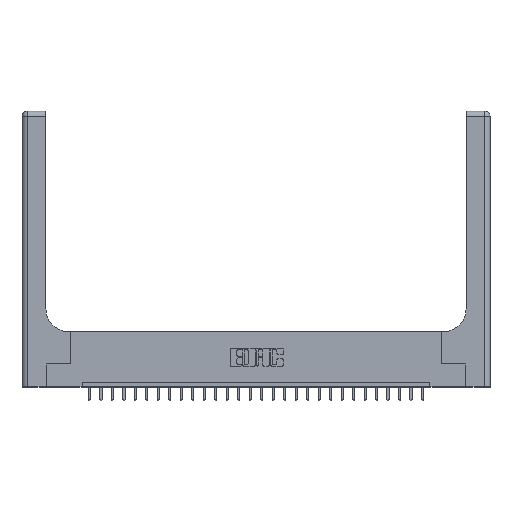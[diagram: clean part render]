
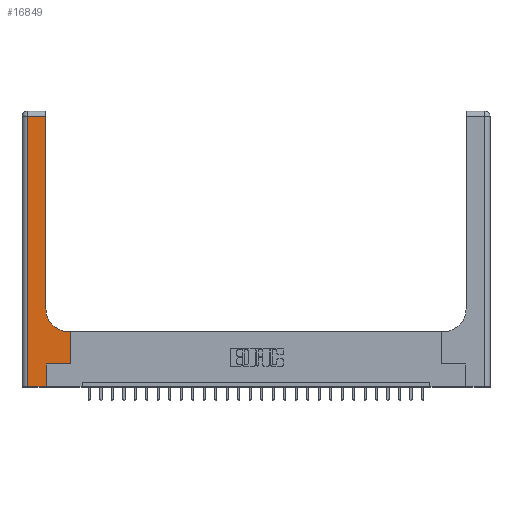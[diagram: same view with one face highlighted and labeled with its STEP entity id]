
A CAD part, top view. The second image highlights one B-rep face of the part: STEP entity #16849.
In plain terms, the highlighted planar face has unit normal (0, 0, 1).
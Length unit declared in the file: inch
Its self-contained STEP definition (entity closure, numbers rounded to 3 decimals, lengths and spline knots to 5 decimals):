
#453 = AXIS2_PLACEMENT_3D ( 'NONE', #2318, #19704, #15861 ) ;
#462 = VECTOR ( 'NONE', #22440, 39.37008 ) ;
#490 = LINE ( 'NONE', #11564, #20848 ) ;
#494 = CARTESIAN_POINT ( 'NONE',  ( 0.528, 0.25, 0.37 ) ) ;
#795 = CARTESIAN_POINT ( 'NONE',  ( 0., 0., 0.37 ) ) ;
#1180 = CARTESIAN_POINT ( 'NONE',  ( 0.265, 0., 0.37 ) ) ;
#1442 = EDGE_CURVE ( 'NONE', #18089, #23932, #17264, .T. ) ;
#1767 = CARTESIAN_POINT ( 'NONE',  ( 0.06, 2.94, 0.37 ) ) ;
#2318 = CARTESIAN_POINT ( 'NONE',  ( 0.51, 0.85, 0.37 ) ) ;
#3366 = EDGE_CURVE ( 'NONE', #8961, #10507, #22909, .T. ) ;
#4182 = ORIENTED_EDGE ( 'NONE', *, *, #21186, .T. ) ;
#6448 = CARTESIAN_POINT ( 'NONE',  ( 0.265, 0.25, 0.37 ) ) ;
#6802 = CARTESIAN_POINT ( 'NONE',  ( 0.51, 0.6, 0.37 ) ) ;
#7119 = VERTEX_POINT ( 'NONE', #1767 ) ;
#7430 = EDGE_CURVE ( 'NONE', #13938, #24035, #20508, .T. ) ;
#8339 = VECTOR ( 'NONE', #15401, 39.37008 ) ;
#8549 = VERTEX_POINT ( 'NONE', #18905 ) ;
#8961 = VERTEX_POINT ( 'NONE', #15860 ) ;
#8978 = CARTESIAN_POINT ( 'NONE',  ( 0.265, 0.25, 0.37 ) ) ;
#8983 = CARTESIAN_POINT ( 'NONE',  ( 0.26, 3., 0.37 ) ) ;
#9111 = ORIENTED_EDGE ( 'NONE', *, *, #1442, .T. ) ;
#9596 = VECTOR ( 'NONE', #21881, 39.37008 ) ;
#9639 = ORIENTED_EDGE ( 'NONE', *, *, #20046, .T. ) ;
#10222 = CARTESIAN_POINT ( 'NONE',  ( 0.528, 0.6, 0.37 ) ) ;
#10507 = VERTEX_POINT ( 'NONE', #8978 ) ;
#11564 = CARTESIAN_POINT ( 'NONE',  ( 0.26, 0.6, 0.37 ) ) ;
#11586 = LINE ( 'NONE', #795, #462 ) ;
#11776 = EDGE_CURVE ( 'NONE', #24035, #18089, #490, .T. ) ;
#12011 = CARTESIAN_POINT ( 'NONE',  ( 0.26, 0.85, 0.37 ) ) ;
#12581 = DIRECTION ( 'NONE',  ( 0., 1., 0. ) ) ;
#12740 = ORIENTED_EDGE ( 'NONE', *, *, #11776, .T. ) ;
#12906 = ORIENTED_EDGE ( 'NONE', *, *, #16806, .T. ) ;
#13363 = EDGE_LOOP ( 'NONE', ( #4182, #18503, #9639, #12906, #24876, #24475, #15937, #12740, #9111 ) ) ;
#13938 = VERTEX_POINT ( 'NONE', #18664 ) ;
#14028 = VECTOR ( 'NONE', #21185, 39.37008 ) ;
#14065 = VECTOR ( 'NONE', #25077, 39.37008 ) ;
#14919 = DIRECTION ( 'NONE',  ( 0., 1., 0. ) ) ;
#15401 = DIRECTION ( 'NONE',  ( 0., -1., 0. ) ) ;
#15860 = CARTESIAN_POINT ( 'NONE',  ( 0.265, 0., 0.37 ) ) ;
#15861 = DIRECTION ( 'NONE',  ( 1., 0., 0. ) ) ;
#15937 = ORIENTED_EDGE ( 'NONE', *, *, #7430, .T. ) ;
#16502 = LINE ( 'NONE', #17098, #14028 ) ;
#16503 = CARTESIAN_POINT ( 'NONE',  ( 0.06, 0., 0.37 ) ) ;
#16806 = EDGE_CURVE ( 'NONE', #17456, #8961, #11586, .T. ) ;
#16849 = ADVANCED_FACE ( 'NONE', ( #19591 ), #22276, .F. ) ;
#17098 = CARTESIAN_POINT ( 'NONE',  ( 0., 2.94, 0.37 ) ) ;
#17264 = CIRCLE ( 'NONE', #453, 0.25 ) ;
#17456 = VERTEX_POINT ( 'NONE', #16503 ) ;
#17487 = EDGE_CURVE ( 'NONE', #8549, #7119, #16502, .T. ) ;
#18089 = VERTEX_POINT ( 'NONE', #6802 ) ;
#18503 = ORIENTED_EDGE ( 'NONE', *, *, #17487, .T. ) ;
#18635 = LINE ( 'NONE', #8983, #24714 ) ;
#18664 = CARTESIAN_POINT ( 'NONE',  ( 0.528, 0.25, 0.37 ) ) ;
#18805 = LINE ( 'NONE', #6448, #9596 ) ;
#18905 = CARTESIAN_POINT ( 'NONE',  ( 0.26, 2.94, 0.37 ) ) ;
#19326 = DIRECTION ( 'NONE',  ( -1., 0., 0. ) ) ;
#19573 = DIRECTION ( 'NONE',  ( -1., 0., 0. ) ) ;
#19591 = FACE_OUTER_BOUND ( 'NONE', #13363, .T. ) ;
#19704 = DIRECTION ( 'NONE',  ( 0., 0., -1. ) ) ;
#20001 = AXIS2_PLACEMENT_3D ( 'NONE', #21372, #23044, #19326 ) ;
#20046 = EDGE_CURVE ( 'NONE', #7119, #17456, #20332, .T. ) ;
#20332 = LINE ( 'NONE', #23146, #8339 ) ;
#20508 = LINE ( 'NONE', #494, #22291 ) ;
#20848 = VECTOR ( 'NONE', #19573, 39.37008 ) ;
#21185 = DIRECTION ( 'NONE',  ( -1., 0., 0. ) ) ;
#21186 = EDGE_CURVE ( 'NONE', #23932, #8549, #18635, .T. ) ;
#21372 = CARTESIAN_POINT ( 'NONE',  ( 0., 3., 0.37 ) ) ;
#21881 = DIRECTION ( 'NONE',  ( 1., 0., 0. ) ) ;
#22276 = PLANE ( 'NONE',  #20001 ) ;
#22291 = VECTOR ( 'NONE', #12581, 39.37008 ) ;
#22440 = DIRECTION ( 'NONE',  ( 1., 0., 0. ) ) ;
#22909 = LINE ( 'NONE', #1180, #14065 ) ;
#23044 = DIRECTION ( 'NONE',  ( 0., 0., -1. ) ) ;
#23146 = CARTESIAN_POINT ( 'NONE',  ( 0.06, 3., 0.37 ) ) ;
#23401 = EDGE_CURVE ( 'NONE', #10507, #13938, #18805, .T. ) ;
#23932 = VERTEX_POINT ( 'NONE', #12011 ) ;
#24035 = VERTEX_POINT ( 'NONE', #10222 ) ;
#24475 = ORIENTED_EDGE ( 'NONE', *, *, #23401, .T. ) ;
#24714 = VECTOR ( 'NONE', #14919, 39.37008 ) ;
#24876 = ORIENTED_EDGE ( 'NONE', *, *, #3366, .T. ) ;
#25077 = DIRECTION ( 'NONE',  ( 0., 1., 0. ) ) ;
